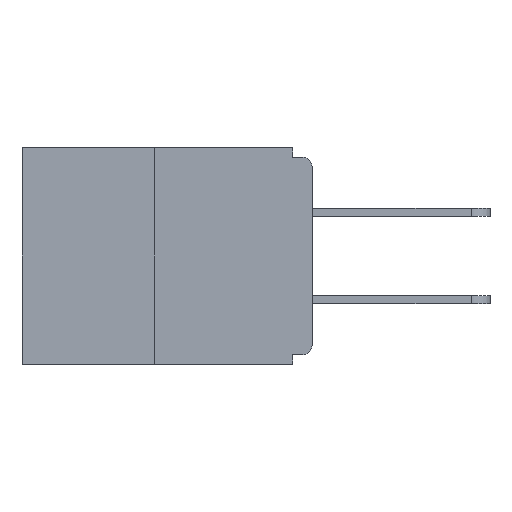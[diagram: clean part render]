
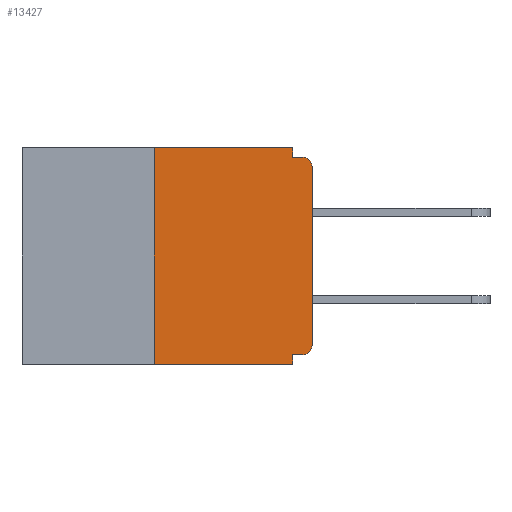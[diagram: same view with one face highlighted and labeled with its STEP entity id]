
A CAD part, left-side view. The second image highlights one B-rep face of the part: STEP entity #13427.
In plain terms, the highlighted planar face has unit normal (-1, 0, 0).
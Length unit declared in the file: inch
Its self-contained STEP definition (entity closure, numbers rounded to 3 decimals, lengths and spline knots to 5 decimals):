
#212 = LINE ( 'NONE', #12977, #18186 ) ;
#684 = CARTESIAN_POINT ( 'NONE',  ( 0., 0., 0. ) ) ;
#1310 = DIRECTION ( 'NONE',  ( 1., 0., 0. ) ) ;
#1358 = EDGE_CURVE ( 'NONE', #16307, #8214, #17436, .T. ) ;
#1368 = VERTEX_POINT ( 'NONE', #6092 ) ;
#1536 = DIRECTION ( 'NONE',  ( 0., 0., -1. ) ) ;
#1635 = VERTEX_POINT ( 'NONE', #2504 ) ;
#1761 = ORIENTED_EDGE ( 'NONE', *, *, #17193, .F. ) ;
#2504 = CARTESIAN_POINT ( 'NONE',  ( 0., 0.031, 0. ) ) ;
#3200 = DIRECTION ( 'NONE',  ( 0., 0., 1. ) ) ;
#3231 = LINE ( 'NONE', #12845, #10543 ) ;
#3264 = DIRECTION ( 'NONE',  ( -1., 0., 0. ) ) ;
#3414 = EDGE_CURVE ( 'NONE', #5867, #17048, #6626, .T. ) ;
#4074 = VECTOR ( 'NONE', #3200, 39.37008 ) ;
#4110 = ORIENTED_EDGE ( 'NONE', *, *, #8495, .F. ) ;
#4320 = EDGE_CURVE ( 'NONE', #5984, #8732, #5441, .T. ) ;
#4572 = CARTESIAN_POINT ( 'NONE',  ( 0., 0.25, 0. ) ) ;
#4702 = CARTESIAN_POINT ( 'NONE',  ( 0., 0.031, -0.343 ) ) ;
#4855 = ORIENTED_EDGE ( 'NONE', *, *, #10787, .F. ) ;
#5063 = AXIS2_PLACEMENT_3D ( 'NONE', #16384, #3264, #6251 ) ;
#5441 = LINE ( 'NONE', #4572, #4074 ) ;
#5708 = DIRECTION ( 'NONE',  ( 0., 1., 0. ) ) ;
#5867 = VERTEX_POINT ( 'NONE', #15742 ) ;
#5984 = VERTEX_POINT ( 'NONE', #18708 ) ;
#6092 = CARTESIAN_POINT ( 'NONE',  ( 0., 0.015, -0.015 ) ) ;
#6183 = LINE ( 'NONE', #7697, #12354 ) ;
#6251 = DIRECTION ( 'NONE',  ( 0., 0., -1. ) ) ;
#6626 = LINE ( 'NONE', #684, #10744 ) ;
#6641 = CARTESIAN_POINT ( 'NONE',  ( 0., 0.031, -0.328 ) ) ;
#6943 = ORIENTED_EDGE ( 'NONE', *, *, #1358, .F. ) ;
#6975 = DIRECTION ( 'NONE',  ( -1., 0., 0. ) ) ;
#7029 = VERTEX_POINT ( 'NONE', #16781 ) ;
#7103 = DIRECTION ( 'NONE',  ( 0., 0., -1. ) ) ;
#7395 = EDGE_LOOP ( 'NONE', ( #16924, #9343, #11442, #6943, #4110, #18020, #10578, #13202, #1761, #4855 ) ) ;
#7697 = CARTESIAN_POINT ( 'NONE',  ( 0., 0.46, -0.343 ) ) ;
#8064 = FACE_OUTER_BOUND ( 'NONE', #7395, .T. ) ;
#8214 = VERTEX_POINT ( 'NONE', #4702 ) ;
#8495 = EDGE_CURVE ( 'NONE', #13732, #16307, #16206, .T. ) ;
#8669 = EDGE_CURVE ( 'NONE', #5984, #8214, #6183, .T. ) ;
#8732 = VERTEX_POINT ( 'NONE', #13340 ) ;
#9158 = VECTOR ( 'NONE', #5708, 39.37008 ) ;
#9343 = ORIENTED_EDGE ( 'NONE', *, *, #4320, .F. ) ;
#9466 = VECTOR ( 'NONE', #13345, 39.37008 ) ;
#9677 = LINE ( 'NONE', #15367, #14427 ) ;
#9683 = DIRECTION ( 'NONE',  ( 0., -1., 0. ) ) ;
#10440 = DIRECTION ( 'NONE',  ( 0., -1., 0. ) ) ;
#10543 = VECTOR ( 'NONE', #9683, 39.37008 ) ;
#10578 = ORIENTED_EDGE ( 'NONE', *, *, #3414, .T. ) ;
#10744 = VECTOR ( 'NONE', #15046, 39.37008 ) ;
#10787 = EDGE_CURVE ( 'NONE', #1635, #7029, #212, .T. ) ;
#11201 = EDGE_CURVE ( 'NONE', #13732, #5867, #12275, .T. ) ;
#11442 = ORIENTED_EDGE ( 'NONE', *, *, #8669, .T. ) ;
#11532 = CARTESIAN_POINT ( 'NONE',  ( 0., 0., -0.328 ) ) ;
#12275 = CIRCLE ( 'NONE', #13473, 0.015 ) ;
#12354 = VECTOR ( 'NONE', #10440, 39.37008 ) ;
#12620 = EDGE_CURVE ( 'NONE', #17048, #1368, #14905, .T. ) ;
#12845 = CARTESIAN_POINT ( 'NONE',  ( 0., 0., -0.015 ) ) ;
#12945 = DIRECTION ( 'NONE',  ( 0., 0., -1. ) ) ;
#12977 = CARTESIAN_POINT ( 'NONE',  ( 0., 0.031, 0. ) ) ;
#13202 = ORIENTED_EDGE ( 'NONE', *, *, #12620, .T. ) ;
#13340 = CARTESIAN_POINT ( 'NONE',  ( 0., 0.25, 0. ) ) ;
#13345 = DIRECTION ( 'NONE',  ( 0., 0., -1. ) ) ;
#13427 = ADVANCED_FACE ( 'NONE', ( #8064 ), #14328, .F. ) ;
#13473 = AXIS2_PLACEMENT_3D ( 'NONE', #15803, #6975, #7103 ) ;
#13732 = VERTEX_POINT ( 'NONE', #18160 ) ;
#13965 = DIRECTION ( 'NONE',  ( 0., -1., 0. ) ) ;
#14328 = PLANE ( 'NONE',  #17920 ) ;
#14427 = VECTOR ( 'NONE', #13965, 39.37008 ) ;
#14905 = CIRCLE ( 'NONE', #5063, 0.015 ) ;
#15046 = DIRECTION ( 'NONE',  ( 0., 0., 1. ) ) ;
#15367 = CARTESIAN_POINT ( 'NONE',  ( 0., 0.46, 0. ) ) ;
#15742 = CARTESIAN_POINT ( 'NONE',  ( 0., 0., -0.313 ) ) ;
#15803 = CARTESIAN_POINT ( 'NONE',  ( 0., 0.015, -0.313 ) ) ;
#16058 = EDGE_CURVE ( 'NONE', #8732, #1635, #9677, .T. ) ;
#16206 = LINE ( 'NONE', #11532, #9158 ) ;
#16276 = CARTESIAN_POINT ( 'NONE',  ( 0., 0.031, -0.343 ) ) ;
#16307 = VERTEX_POINT ( 'NONE', #6641 ) ;
#16384 = CARTESIAN_POINT ( 'NONE',  ( 0., 0.015, -0.03 ) ) ;
#16781 = CARTESIAN_POINT ( 'NONE',  ( 0., 0.031, -0.015 ) ) ;
#16815 = CARTESIAN_POINT ( 'NONE',  ( 0., 0., -0.03 ) ) ;
#16924 = ORIENTED_EDGE ( 'NONE', *, *, #16058, .F. ) ;
#17048 = VERTEX_POINT ( 'NONE', #16815 ) ;
#17193 = EDGE_CURVE ( 'NONE', #7029, #1368, #3231, .T. ) ;
#17436 = LINE ( 'NONE', #16276, #9466 ) ;
#17920 = AXIS2_PLACEMENT_3D ( 'NONE', #18711, #1310, #12945 ) ;
#18020 = ORIENTED_EDGE ( 'NONE', *, *, #11201, .T. ) ;
#18160 = CARTESIAN_POINT ( 'NONE',  ( 0., 0.015, -0.328 ) ) ;
#18186 = VECTOR ( 'NONE', #1536, 39.37008 ) ;
#18708 = CARTESIAN_POINT ( 'NONE',  ( 0., 0.25, -0.343 ) ) ;
#18711 = CARTESIAN_POINT ( 'NONE',  ( 0., 0.46, 0. ) ) ;
